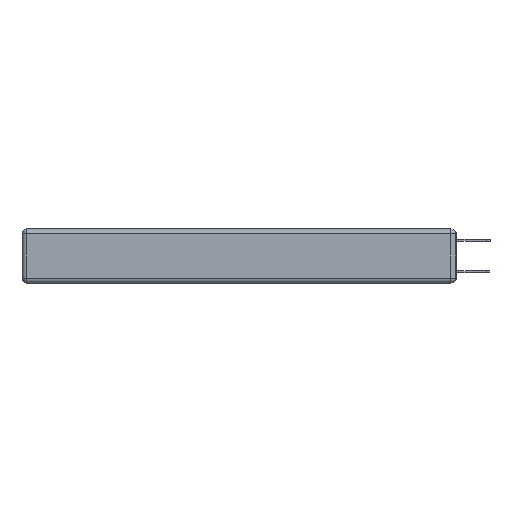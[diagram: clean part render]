
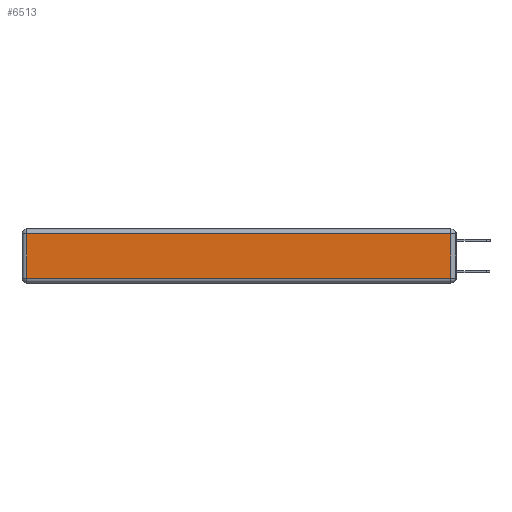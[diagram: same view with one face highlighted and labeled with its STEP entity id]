
A CAD part, left-side view. The second image highlights one B-rep face of the part: STEP entity #6513.
In plain terms, the highlighted planar face has unit normal (-1, 0, 0).
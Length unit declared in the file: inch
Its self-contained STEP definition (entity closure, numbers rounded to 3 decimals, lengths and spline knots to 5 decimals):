
#253 = DIRECTION ( 'NONE',  ( 0., 0., -1. ) ) ;
#342 = ORIENTED_EDGE ( 'NONE', *, *, #2787, .T. ) ;
#541 = CARTESIAN_POINT ( 'NONE',  ( 0., 0.03, -0.343 ) ) ;
#611 = DIRECTION ( 'NONE',  ( 0., 0., 1. ) ) ;
#713 = VERTEX_POINT ( 'NONE', #10984 ) ;
#1420 = VERTEX_POINT ( 'NONE', #2215 ) ;
#1545 = FACE_OUTER_BOUND ( 'NONE', #9991, .T. ) ;
#1680 = PLANE ( 'NONE',  #10689 ) ;
#1885 = LINE ( 'NONE', #6134, #5807 ) ;
#2215 = CARTESIAN_POINT ( 'NONE',  ( 0., 0.03, -0.313 ) ) ;
#2787 = EDGE_CURVE ( 'NONE', #6015, #1420, #8487, .T. ) ;
#3435 = CARTESIAN_POINT ( 'NONE',  ( 0., 0., -0.313 ) ) ;
#4605 = CARTESIAN_POINT ( 'NONE',  ( 0., 2.72, -0.313 ) ) ;
#5142 = DIRECTION ( 'NONE',  ( 0., 1., 0. ) ) ;
#5149 = VECTOR ( 'NONE', #5800, 39.37008 ) ;
#5593 = ORIENTED_EDGE ( 'NONE', *, *, #6595, .T. ) ;
#5800 = DIRECTION ( 'NONE',  ( 0., 0., 1. ) ) ;
#5807 = VECTOR ( 'NONE', #5142, 39.37008 ) ;
#6015 = VERTEX_POINT ( 'NONE', #4605 ) ;
#6134 = CARTESIAN_POINT ( 'NONE',  ( 0., 2.75, -0.03 ) ) ;
#6259 = ORIENTED_EDGE ( 'NONE', *, *, #9605, .T. ) ;
#6513 = ADVANCED_FACE ( 'NONE', ( #1545 ), #1680, .T. ) ;
#6595 = EDGE_CURVE ( 'NONE', #1420, #713, #7835, .T. ) ;
#6742 = EDGE_CURVE ( 'NONE', #8176, #6015, #7454, .T. ) ;
#7454 = LINE ( 'NONE', #10530, #10476 ) ;
#7835 = LINE ( 'NONE', #541, #5149 ) ;
#8176 = VERTEX_POINT ( 'NONE', #9158 ) ;
#8487 = LINE ( 'NONE', #3435, #12142 ) ;
#8701 = ORIENTED_EDGE ( 'NONE', *, *, #6742, .T. ) ;
#9158 = CARTESIAN_POINT ( 'NONE',  ( 0., 2.72, -0.03 ) ) ;
#9605 = EDGE_CURVE ( 'NONE', #713, #8176, #1885, .T. ) ;
#9991 = EDGE_LOOP ( 'NONE', ( #342, #5593, #6259, #8701 ) ) ;
#10476 = VECTOR ( 'NONE', #253, 39.37008 ) ;
#10530 = CARTESIAN_POINT ( 'NONE',  ( 0., 2.72, -0.343 ) ) ;
#10689 = AXIS2_PLACEMENT_3D ( 'NONE', #11034, #12042, #611 ) ;
#10984 = CARTESIAN_POINT ( 'NONE',  ( 0., 0.03, -0.03 ) ) ;
#11034 = CARTESIAN_POINT ( 'NONE',  ( 0., 0., -0.343 ) ) ;
#12042 = DIRECTION ( 'NONE',  ( -1., 0., 0. ) ) ;
#12142 = VECTOR ( 'NONE', #12559, 39.37008 ) ;
#12559 = DIRECTION ( 'NONE',  ( 0., -1., 0. ) ) ;
